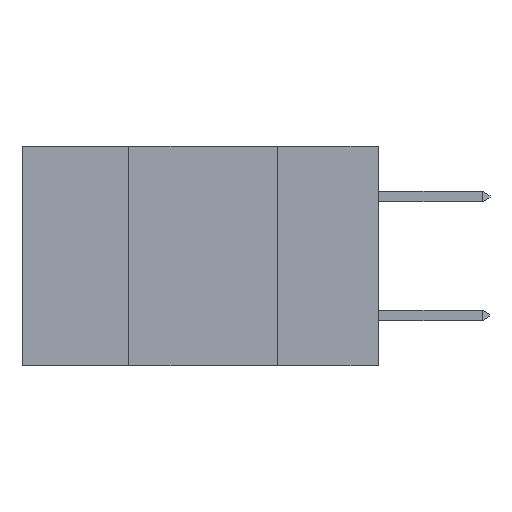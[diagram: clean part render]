
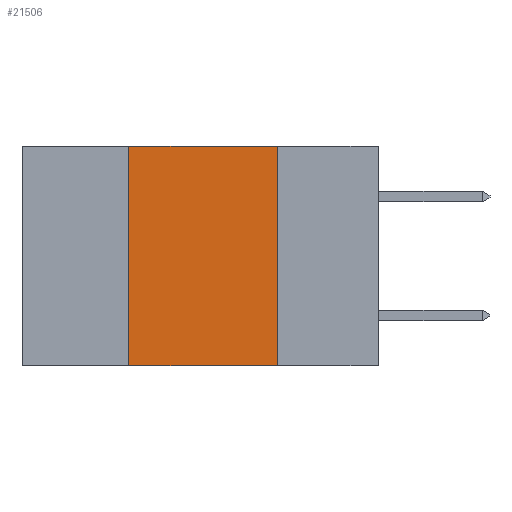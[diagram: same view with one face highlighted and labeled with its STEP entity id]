
A CAD part, left-side view. The second image highlights one B-rep face of the part: STEP entity #21506.
In plain terms, the highlighted planar face has unit normal (-1, 0, 0).
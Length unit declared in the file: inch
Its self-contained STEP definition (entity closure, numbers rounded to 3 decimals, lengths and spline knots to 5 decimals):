
#392 = ORIENTED_EDGE ( 'NONE', *, *, #14855, .F. ) ;
#1253 = DIRECTION ( 'NONE',  ( 0., 0., -1. ) ) ;
#2179 = CARTESIAN_POINT ( 'NONE',  ( 0., 0.42, 0. ) ) ;
#2717 = LINE ( 'NONE', #2179, #18381 ) ;
#2849 = VERTEX_POINT ( 'NONE', #12814 ) ;
#2897 = LINE ( 'NONE', #21996, #7747 ) ;
#3271 = CARTESIAN_POINT ( 'NONE',  ( 0., 0.6, 0. ) ) ;
#4271 = DIRECTION ( 'NONE',  ( 0., 0., 1. ) ) ;
#5847 = VECTOR ( 'NONE', #23057, 39.37008 ) ;
#7747 = VECTOR ( 'NONE', #11936, 39.37008 ) ;
#9303 = ORIENTED_EDGE ( 'NONE', *, *, #12184, .T. ) ;
#10545 = CARTESIAN_POINT ( 'NONE',  ( 0., 0.42, 0. ) ) ;
#10617 = VERTEX_POINT ( 'NONE', #12110 ) ;
#10916 = EDGE_LOOP ( 'NONE', ( #23112, #16226, #392, #9303 ) ) ;
#11936 = DIRECTION ( 'NONE',  ( 0., 0., -1. ) ) ;
#12110 = CARTESIAN_POINT ( 'NONE',  ( 0., 0.17, 0. ) ) ;
#12184 = EDGE_CURVE ( 'NONE', #17841, #2849, #16314, .T. ) ;
#12814 = CARTESIAN_POINT ( 'NONE',  ( 0., 0.17, -0.37 ) ) ;
#13575 = DIRECTION ( 'NONE',  ( 1., 0., 0. ) ) ;
#14855 = EDGE_CURVE ( 'NONE', #17841, #19544, #2717, .T. ) ;
#16226 = ORIENTED_EDGE ( 'NONE', *, *, #22635, .F. ) ;
#16314 = LINE ( 'NONE', #16512, #26354 ) ;
#16512 = CARTESIAN_POINT ( 'NONE',  ( 0., 0.6, -0.37 ) ) ;
#17707 = FACE_OUTER_BOUND ( 'NONE', #10916, .T. ) ;
#17841 = VERTEX_POINT ( 'NONE', #19248 ) ;
#18381 = VECTOR ( 'NONE', #4271, 39.37008 ) ;
#18556 = DIRECTION ( 'NONE',  ( 0., -1., 0. ) ) ;
#19248 = CARTESIAN_POINT ( 'NONE',  ( 0., 0.42, -0.37 ) ) ;
#19544 = VERTEX_POINT ( 'NONE', #10545 ) ;
#20695 = AXIS2_PLACEMENT_3D ( 'NONE', #3271, #13575, #1253 ) ;
#21033 = CARTESIAN_POINT ( 'NONE',  ( 0., 0.6, 0. ) ) ;
#21506 = ADVANCED_FACE ( 'NONE', ( #17707 ), #25635, .F. ) ;
#21996 = CARTESIAN_POINT ( 'NONE',  ( 0., 0.17, 0. ) ) ;
#22635 = EDGE_CURVE ( 'NONE', #19544, #10617, #22685, .T. ) ;
#22685 = LINE ( 'NONE', #21033, #5847 ) ;
#22978 = EDGE_CURVE ( 'NONE', #10617, #2849, #2897, .T. ) ;
#23057 = DIRECTION ( 'NONE',  ( 0., -1., 0. ) ) ;
#23112 = ORIENTED_EDGE ( 'NONE', *, *, #22978, .F. ) ;
#25635 = PLANE ( 'NONE',  #20695 ) ;
#26354 = VECTOR ( 'NONE', #18556, 39.37008 ) ;
